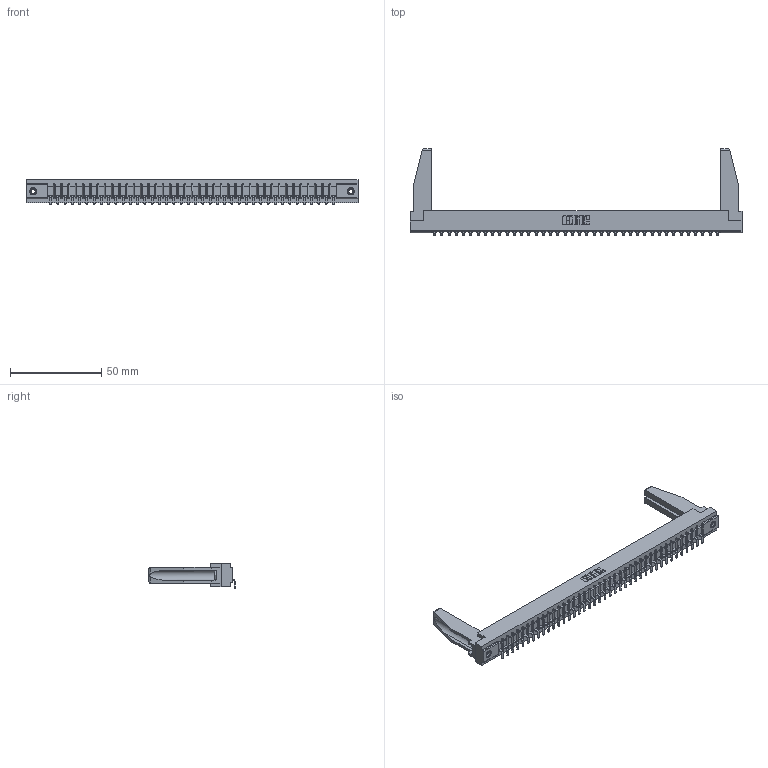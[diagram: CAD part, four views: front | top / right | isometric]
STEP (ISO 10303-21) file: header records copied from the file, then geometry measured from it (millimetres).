
FILE_DESCRIPTION (( 'STEP AP203' ), '1' );
FILE_NAME ('307-040-553-178.STEP', '2019-09-05T10:36:14', ( '' ), ( '' ), 'SwSTEP 2.0', 'SolidWorks 2016', '' );
FILE_SCHEMA (( 'CONFIG_CONTROL_DESIGN' ));
Length unit declared in the file: inch
Products named in the file (5): 307-220-078; 307 Part_.156 Dia Mounting Holes; 307-290-002_553; 345-250-001_345-250-001-102; 307-040-553-178
Assembly tree (45 placements, depth 2):
  307-040-553-178
    307 Part_.156 Dia Mounting Holes
    307-290-002_553  x40
    307-220-078  x2
    345-250-001_345-250-001-102  x2
Bounding box: 181.51 x 47.03 x 13.5 mm (x, y, z)
Volume: 23401.9 mm3; surface area: 28178.4 mm2
Topology: 45 solids, 45 shells, 3409 faces, 10413 edges, 6822 vertices
Faces by surface type: plane 2034, cylinder 1277, sphere 82, cone 12, torus 4
Entity records: 37831 total; most frequent: CARTESIAN_POINT 6382, ORIENTED_EDGE 6328, DIRECTION 6158, EDGE_CURVE 3164, LINE 2426, VECTOR 2426, VERTEX_POINT 2048, AXIS2_PLACEMENT_3D 1866
